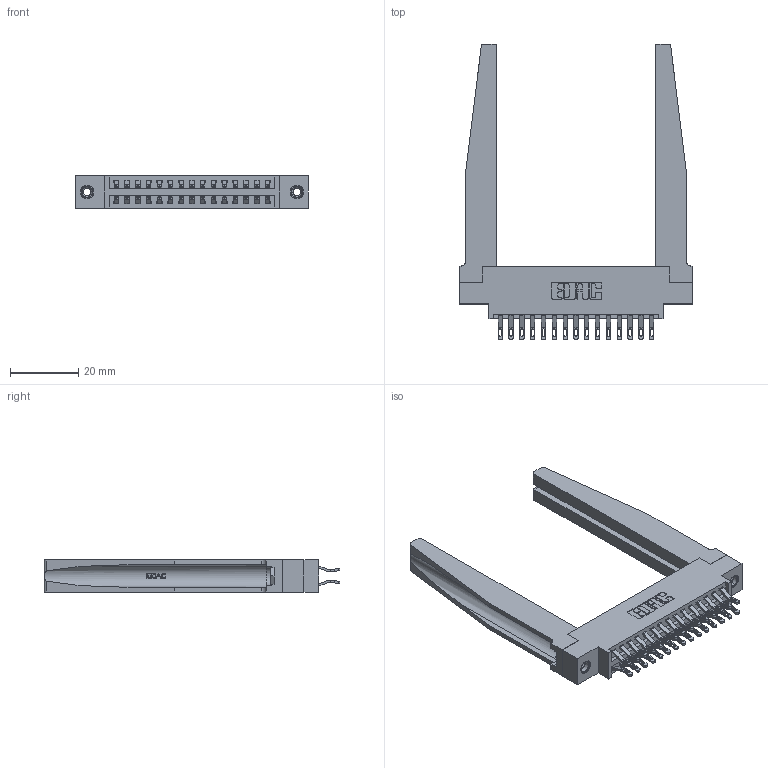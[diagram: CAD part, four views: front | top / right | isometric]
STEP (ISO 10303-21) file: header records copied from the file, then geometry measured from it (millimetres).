
FILE_DESCRIPTION (( 'STEP AP203' ), '1' );
FILE_NAME ('346-030-555-878.STEP', '2022-05-19T16:48:58', ( '' ), ( '' ), 'SwSTEP 2.0', 'SolidWorks 2020', '' );
FILE_SCHEMA (( 'CONFIG_CONTROL_DESIGN' ));
Length unit declared in the file: inch
Products named in the file (5): 346-030-555-878; 345-250-001_345-250-001-102; 346 Part_0.170 Offset - 0.156 Dia-TH; 345-292-001_555 Tail; 346-220-078_345-220-078
Assembly tree (35 placements, depth 2):
  346-030-555-878
    346 Part_0.170 Offset - 0.156 Dia-TH
    345-292-001_555 Tail  x30
    346-220-078_345-220-078  x2
    345-250-001_345-250-001-102  x2
Bounding box: 68.2 x 86.74 x 9.4 mm (x, y, z)
Volume: 13263.7 mm3; surface area: 15372.7 mm2
Topology: 35 solids, 35 shells, 2114 faces, 6475 edges, 4306 vertices
Faces by surface type: plane 1226, cylinder 836, bspline 36, cone 12, torus 4
Entity records: 19046 total; most frequent: CARTESIAN_POINT 4155, ORIENTED_EDGE 2946, DIRECTION 2667, EDGE_CURVE 1473, VECTOR 1167, LINE 1167, VERTEX_POINT 976, AXIS2_PLACEMENT_3D 750
